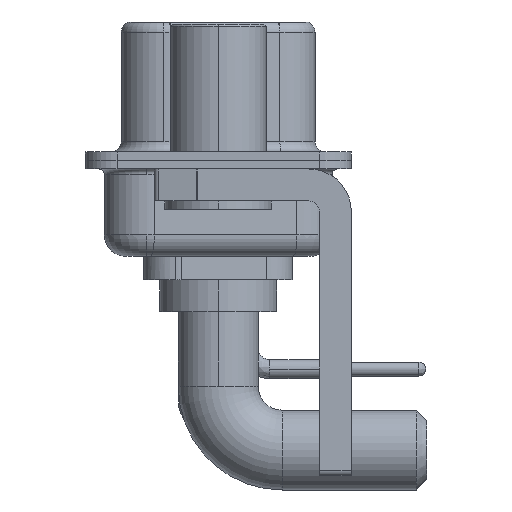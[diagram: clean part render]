
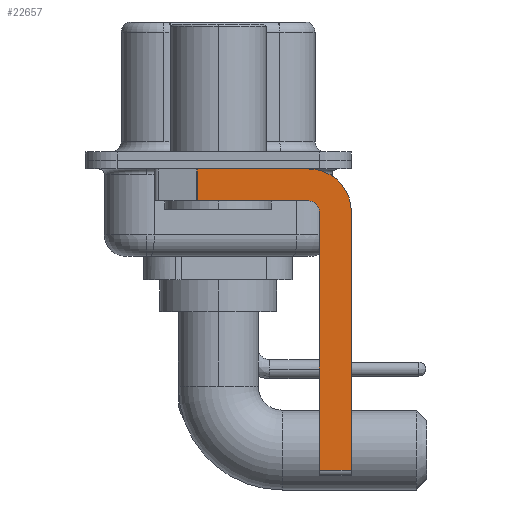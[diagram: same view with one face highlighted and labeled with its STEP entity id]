
A CAD part, left-side view. The second image highlights one B-rep face of the part: STEP entity #22657.
In plain terms, the highlighted planar face has unit normal (-1, 0, 0).
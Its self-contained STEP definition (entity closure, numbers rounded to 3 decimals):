
#1093 = AXIS2_PLACEMENT_3D ( 'NONE', #27066, #14308, #21061 ) ;
#1291 = LINE ( 'NONE', #9518, #25350 ) ;
#1302 = DIRECTION ( 'NONE',  ( 0., -1., 0. ) ) ;
#1843 = LINE ( 'NONE', #5949, #5366 ) ;
#2199 = EDGE_CURVE ( 'NONE', #23018, #18678, #7689, .T. ) ;
#2408 = ORIENTED_EDGE ( 'NONE', *, *, #25756, .F. ) ;
#2637 = VERTEX_POINT ( 'NONE', #21321 ) ;
#3062 = CARTESIAN_POINT ( 'NONE',  ( -2.9, 0.978, -1.9 ) ) ;
#3413 = PLANE ( 'NONE',  #1093 ) ;
#3521 = CARTESIAN_POINT ( 'NONE',  ( -2.9, -4.25, -2.4 ) ) ;
#5355 = CARTESIAN_POINT ( 'NONE',  ( -2.9, -4.75, -14.55 ) ) ;
#5366 = VECTOR ( 'NONE', #19041, 1000. ) ;
#5949 = CARTESIAN_POINT ( 'NONE',  ( -2.9, 0.978, -1.9 ) ) ;
#6587 = VECTOR ( 'NONE', #19709, 1000. ) ;
#6870 = ORIENTED_EDGE ( 'NONE', *, *, #18720, .F. ) ;
#7151 = ORIENTED_EDGE ( 'NONE', *, *, #24473, .F. ) ;
#7689 = LINE ( 'NONE', #20795, #9599 ) ;
#7785 = DIRECTION ( 'NONE',  ( 1., 0., 0. ) ) ;
#9048 = DIRECTION ( 'NONE',  ( -1., 0., 0. ) ) ;
#9465 = CARTESIAN_POINT ( 'NONE',  ( -2.9, 0.978, -0.4 ) ) ;
#9518 = CARTESIAN_POINT ( 'NONE',  ( -2.9, -4.25, -1.9 ) ) ;
#9599 = VECTOR ( 'NONE', #1302, 1000. ) ;
#9791 = DIRECTION ( 'NONE',  ( 0., -1., 0. ) ) ;
#10079 = DIRECTION ( 'NONE',  ( 0., 1., 0. ) ) ;
#10749 = DIRECTION ( 'NONE',  ( 0., 0., -1. ) ) ;
#11909 = LINE ( 'NONE', #20622, #20683 ) ;
#12476 = CARTESIAN_POINT ( 'NONE',  ( -2.9, -6.25, -2.4 ) ) ;
#12612 = LINE ( 'NONE', #12476, #21882 ) ;
#13001 = AXIS2_PLACEMENT_3D ( 'NONE', #22294, #9048, #26596 ) ;
#13277 = CARTESIAN_POINT ( 'NONE',  ( -2.9, -4.75, -14.8 ) ) ;
#13355 = ORIENTED_EDGE ( 'NONE', *, *, #15278, .T. ) ;
#13371 = EDGE_CURVE ( 'NONE', #24411, #2637, #19566, .T. ) ;
#14170 = FACE_OUTER_BOUND ( 'NONE', #17560, .T. ) ;
#14280 = EDGE_CURVE ( 'NONE', #26376, #26594, #1291, .T. ) ;
#14308 = DIRECTION ( 'NONE',  ( 1., 0., 0. ) ) ;
#14965 = ORIENTED_EDGE ( 'NONE', *, *, #26102, .F. ) ;
#15261 = CARTESIAN_POINT ( 'NONE',  ( -2.9, -4.25, -1.9 ) ) ;
#15278 = EDGE_CURVE ( 'NONE', #18931, #26594, #1843, .T. ) ;
#16301 = ORIENTED_EDGE ( 'NONE', *, *, #14280, .F. ) ;
#16818 = ORIENTED_EDGE ( 'NONE', *, *, #2199, .T. ) ;
#17560 = EDGE_LOOP ( 'NONE', ( #2408, #13355, #16301, #14965, #7151, #16818, #6870, #26139 ) ) ;
#18273 = CARTESIAN_POINT ( 'NONE',  ( -2.9, -4.75, -2.4 ) ) ;
#18590 = DIRECTION ( 'NONE',  ( 0., 0., -1. ) ) ;
#18678 = VERTEX_POINT ( 'NONE', #28038 ) ;
#18720 = EDGE_CURVE ( 'NONE', #2637, #18678, #12612, .T. ) ;
#18931 = VERTEX_POINT ( 'NONE', #9465 ) ;
#19041 = DIRECTION ( 'NONE',  ( 0., 0., -1. ) ) ;
#19566 = CIRCLE ( 'NONE', #25520, 2. ) ;
#19709 = DIRECTION ( 'NONE',  ( 0., 0., 1. ) ) ;
#19854 = LINE ( 'NONE', #13277, #6587 ) ;
#20622 = CARTESIAN_POINT ( 'NONE',  ( -2.9, 3., -0.4 ) ) ;
#20683 = VECTOR ( 'NONE', #9791, 1000. ) ;
#20795 = CARTESIAN_POINT ( 'NONE',  ( -2.9, -4.25, -14.55 ) ) ;
#21061 = DIRECTION ( 'NONE',  ( 0., 0., -1. ) ) ;
#21321 = CARTESIAN_POINT ( 'NONE',  ( -2.9, -6.25, -2.4 ) ) ;
#21882 = VECTOR ( 'NONE', #10749, 1000. ) ;
#22294 = CARTESIAN_POINT ( 'NONE',  ( -2.9, -4.25, -2.4 ) ) ;
#22592 = CIRCLE ( 'NONE', #13001, 0.5 ) ;
#22657 = ADVANCED_FACE ( 'NONE', ( #14170 ), #3413, .F. ) ;
#23018 = VERTEX_POINT ( 'NONE', #5355 ) ;
#23390 = VERTEX_POINT ( 'NONE', #18273 ) ;
#24411 = VERTEX_POINT ( 'NONE', #25737 ) ;
#24473 = EDGE_CURVE ( 'NONE', #23018, #23390, #19854, .T. ) ;
#25350 = VECTOR ( 'NONE', #10079, 1000. ) ;
#25520 = AXIS2_PLACEMENT_3D ( 'NONE', #3521, #7785, #18590 ) ;
#25737 = CARTESIAN_POINT ( 'NONE',  ( -2.9, -4.25, -0.4 ) ) ;
#25756 = EDGE_CURVE ( 'NONE', #18931, #24411, #11909, .T. ) ;
#26102 = EDGE_CURVE ( 'NONE', #23390, #26376, #22592, .T. ) ;
#26139 = ORIENTED_EDGE ( 'NONE', *, *, #13371, .F. ) ;
#26376 = VERTEX_POINT ( 'NONE', #15261 ) ;
#26594 = VERTEX_POINT ( 'NONE', #3062 ) ;
#26596 = DIRECTION ( 'NONE',  ( 0., 0., 1. ) ) ;
#27066 = CARTESIAN_POINT ( 'NONE',  ( -2.9, -4.25, -2.4 ) ) ;
#28038 = CARTESIAN_POINT ( 'NONE',  ( -2.9, -6.25, -14.55 ) ) ;
